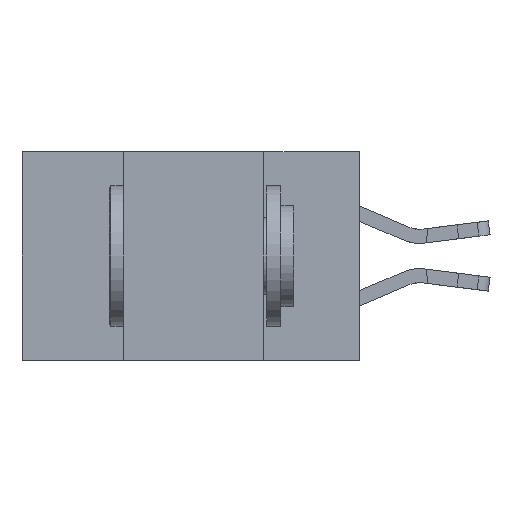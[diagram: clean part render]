
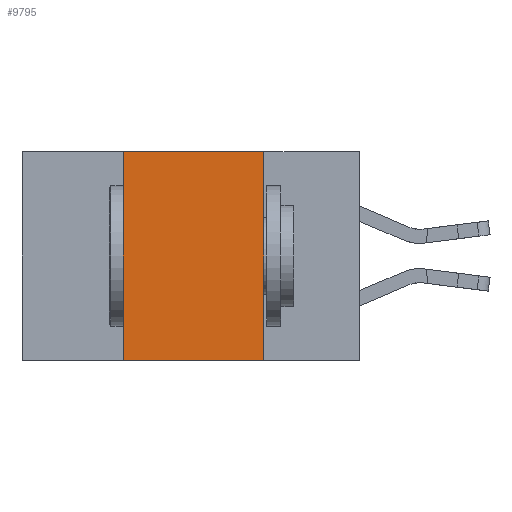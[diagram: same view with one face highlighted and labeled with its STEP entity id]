
A CAD part, left-side view. The second image highlights one B-rep face of the part: STEP entity #9795.
In plain terms, the highlighted planar face has unit normal (-1, 0, 0).
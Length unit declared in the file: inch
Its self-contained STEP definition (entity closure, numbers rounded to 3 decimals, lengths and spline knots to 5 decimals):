
#171 = EDGE_CURVE ( 'NONE', #21419, #18179, #16033, .T. ) ;
#684 = VECTOR ( 'NONE', #1187, 39.37008 ) ;
#1159 = DIRECTION ( 'NONE',  ( 0., 0., -1. ) ) ;
#1187 = DIRECTION ( 'NONE',  ( 0., -1., 0. ) ) ;
#1239 = CARTESIAN_POINT ( 'NONE',  ( 0., 0.42, -0.37 ) ) ;
#3049 = FACE_OUTER_BOUND ( 'NONE', #24001, .T. ) ;
#4108 = CARTESIAN_POINT ( 'NONE',  ( 0., 0.17, -0.37 ) ) ;
#4336 = EDGE_CURVE ( 'NONE', #5702, #14407, #21185, .T. ) ;
#4667 = CARTESIAN_POINT ( 'NONE',  ( 0., 0.17, 0. ) ) ;
#5640 = LINE ( 'NONE', #21960, #684 ) ;
#5702 = VERTEX_POINT ( 'NONE', #11693 ) ;
#5854 = DIRECTION ( 'NONE',  ( 0., 0., 1. ) ) ;
#5874 = EDGE_CURVE ( 'NONE', #21419, #14407, #22356, .T. ) ;
#7217 = VECTOR ( 'NONE', #5854, 39.37008 ) ;
#7318 = VECTOR ( 'NONE', #22058, 39.37008 ) ;
#8456 = ORIENTED_EDGE ( 'NONE', *, *, #13839, .F. ) ;
#9795 = ADVANCED_FACE ( 'NONE', ( #3049 ), #23618, .F. ) ;
#9878 = ORIENTED_EDGE ( 'NONE', *, *, #5874, .T. ) ;
#10445 = CARTESIAN_POINT ( 'NONE',  ( 0., 0.6, -0.37 ) ) ;
#11693 = CARTESIAN_POINT ( 'NONE',  ( 0., 0.17, 0. ) ) ;
#12146 = ORIENTED_EDGE ( 'NONE', *, *, #4336, .F. ) ;
#12230 = ORIENTED_EDGE ( 'NONE', *, *, #171, .F. ) ;
#13839 = EDGE_CURVE ( 'NONE', #18179, #5702, #5640, .T. ) ;
#14407 = VERTEX_POINT ( 'NONE', #4108 ) ;
#14956 = AXIS2_PLACEMENT_3D ( 'NONE', #21726, #23541, #19739 ) ;
#16033 = LINE ( 'NONE', #16949, #7217 ) ;
#16949 = CARTESIAN_POINT ( 'NONE',  ( 0., 0.42, 0. ) ) ;
#18179 = VERTEX_POINT ( 'NONE', #19215 ) ;
#19108 = VECTOR ( 'NONE', #1159, 39.37008 ) ;
#19215 = CARTESIAN_POINT ( 'NONE',  ( 0., 0.42, 0. ) ) ;
#19739 = DIRECTION ( 'NONE',  ( 0., 0., -1. ) ) ;
#21185 = LINE ( 'NONE', #4667, #19108 ) ;
#21419 = VERTEX_POINT ( 'NONE', #1239 ) ;
#21726 = CARTESIAN_POINT ( 'NONE',  ( 0., 0.6, 0. ) ) ;
#21960 = CARTESIAN_POINT ( 'NONE',  ( 0., 0.6, 0. ) ) ;
#22058 = DIRECTION ( 'NONE',  ( 0., -1., 0. ) ) ;
#22356 = LINE ( 'NONE', #10445, #7318 ) ;
#23541 = DIRECTION ( 'NONE',  ( 1., 0., 0. ) ) ;
#23618 = PLANE ( 'NONE',  #14956 ) ;
#24001 = EDGE_LOOP ( 'NONE', ( #12146, #8456, #12230, #9878 ) ) ;
